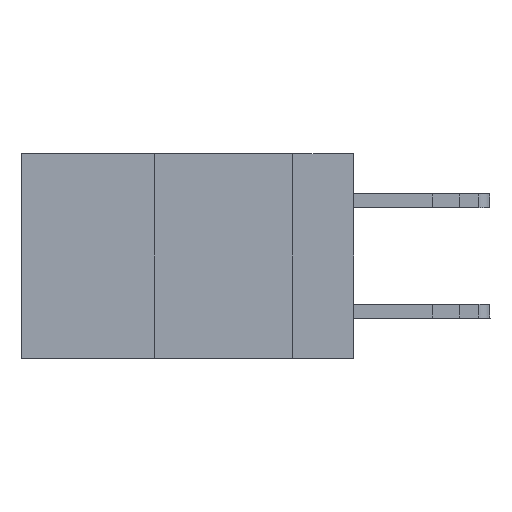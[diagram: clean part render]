
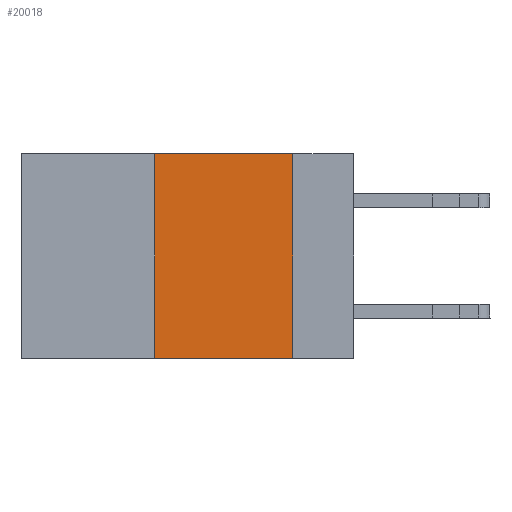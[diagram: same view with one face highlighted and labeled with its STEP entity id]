
A CAD part, left-side view. The second image highlights one B-rep face of the part: STEP entity #20018.
In plain terms, the highlighted planar face has unit normal (-1, 0, 0).
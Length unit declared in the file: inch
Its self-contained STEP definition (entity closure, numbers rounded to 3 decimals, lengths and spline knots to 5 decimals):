
#296 = LINE ( 'NONE', #17963, #13185 ) ;
#877 = EDGE_CURVE ( 'NONE', #17468, #22185, #296, .T. ) ;
#1810 = FACE_OUTER_BOUND ( 'NONE', #11873, .T. ) ;
#4259 = DIRECTION ( 'NONE',  ( 0., 0., -1. ) ) ;
#5907 = PLANE ( 'NONE',  #7084 ) ;
#7084 = AXIS2_PLACEMENT_3D ( 'NONE', #8322, #21933, #10513 ) ;
#7926 = LINE ( 'NONE', #26932, #14371 ) ;
#8123 = EDGE_CURVE ( 'NONE', #22113, #22185, #12598, .T. ) ;
#8322 = CARTESIAN_POINT ( 'NONE',  ( 0., 0.6, 0. ) ) ;
#8452 = DIRECTION ( 'NONE',  ( 0., -1., 0. ) ) ;
#8613 = EDGE_CURVE ( 'NONE', #22113, #12066, #16568, .T. ) ;
#10513 = DIRECTION ( 'NONE',  ( 0., 0., -1. ) ) ;
#11873 = EDGE_LOOP ( 'NONE', ( #22151, #25444, #27825, #20926 ) ) ;
#12058 = CARTESIAN_POINT ( 'NONE',  ( 0., 0.36, 0. ) ) ;
#12066 = VERTEX_POINT ( 'NONE', #12058 ) ;
#12598 = LINE ( 'NONE', #19912, #16534 ) ;
#12950 = DIRECTION ( 'NONE',  ( 0., -1., 0. ) ) ;
#13185 = VECTOR ( 'NONE', #4259, 39.37008 ) ;
#14371 = VECTOR ( 'NONE', #8452, 39.37008 ) ;
#15115 = VECTOR ( 'NONE', #18774, 39.37008 ) ;
#16534 = VECTOR ( 'NONE', #12950, 39.37008 ) ;
#16568 = LINE ( 'NONE', #23324, #15115 ) ;
#17468 = VERTEX_POINT ( 'NONE', #24498 ) ;
#17963 = CARTESIAN_POINT ( 'NONE',  ( 0., 0.11, 0. ) ) ;
#18774 = DIRECTION ( 'NONE',  ( 0., 0., 1. ) ) ;
#19912 = CARTESIAN_POINT ( 'NONE',  ( 0., 0.6, -0.37 ) ) ;
#20018 = ADVANCED_FACE ( 'NONE', ( #1810 ), #5907, .F. ) ;
#20926 = ORIENTED_EDGE ( 'NONE', *, *, #8123, .T. ) ;
#21933 = DIRECTION ( 'NONE',  ( 1., 0., 0. ) ) ;
#22113 = VERTEX_POINT ( 'NONE', #24536 ) ;
#22151 = ORIENTED_EDGE ( 'NONE', *, *, #877, .F. ) ;
#22185 = VERTEX_POINT ( 'NONE', #24741 ) ;
#23324 = CARTESIAN_POINT ( 'NONE',  ( 0., 0.36, 0. ) ) ;
#24498 = CARTESIAN_POINT ( 'NONE',  ( 0., 0.11, 0. ) ) ;
#24536 = CARTESIAN_POINT ( 'NONE',  ( 0., 0.36, -0.37 ) ) ;
#24741 = CARTESIAN_POINT ( 'NONE',  ( 0., 0.11, -0.37 ) ) ;
#25444 = ORIENTED_EDGE ( 'NONE', *, *, #25893, .F. ) ;
#25893 = EDGE_CURVE ( 'NONE', #12066, #17468, #7926, .T. ) ;
#26932 = CARTESIAN_POINT ( 'NONE',  ( 0., 0.6, 0. ) ) ;
#27825 = ORIENTED_EDGE ( 'NONE', *, *, #8613, .F. ) ;
